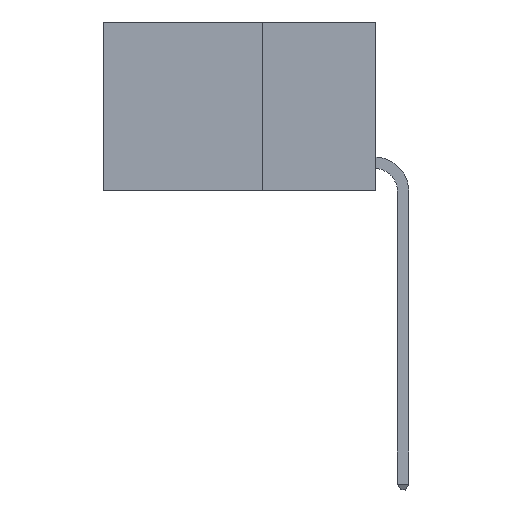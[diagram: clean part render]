
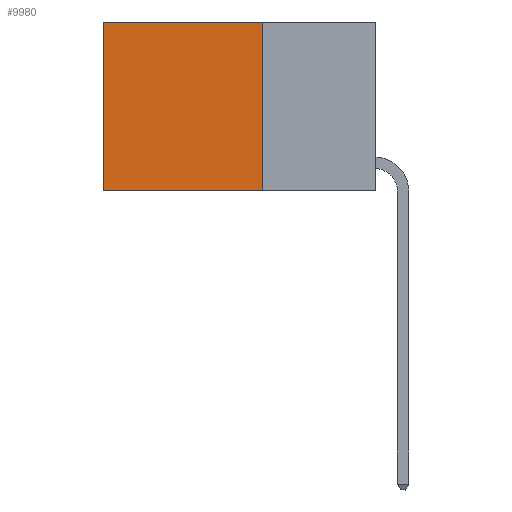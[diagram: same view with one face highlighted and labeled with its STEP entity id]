
A CAD part, left-side view. The second image highlights one B-rep face of the part: STEP entity #9980.
In plain terms, the highlighted planar face has unit normal (-1, 0, 0).
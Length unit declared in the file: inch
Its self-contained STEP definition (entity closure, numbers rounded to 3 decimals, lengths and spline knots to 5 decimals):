
#151 = ORIENTED_EDGE ( 'NONE', *, *, #3147, .F. ) ;
#350 = CARTESIAN_POINT ( 'NONE',  ( 0.2625, 0.25, -0.37 ) ) ;
#487 = VECTOR ( 'NONE', #7793, 39.37008 ) ;
#521 = CARTESIAN_POINT ( 'NONE',  ( 0.2625, 0.6, 0. ) ) ;
#723 = ORIENTED_EDGE ( 'NONE', *, *, #13557, .T. ) ;
#1414 = EDGE_LOOP ( 'NONE', ( #4210, #13328, #151, #723 ) ) ;
#2627 = CARTESIAN_POINT ( 'NONE',  ( 0.2625, 0.25, 0. ) ) ;
#3147 = EDGE_CURVE ( 'NONE', #5640, #12614, #14570, .T. ) ;
#3523 = CARTESIAN_POINT ( 'NONE',  ( 0.2625, 0.6, 0. ) ) ;
#3679 = CARTESIAN_POINT ( 'NONE',  ( 0.2625, 0.25, 0. ) ) ;
#3806 = FACE_OUTER_BOUND ( 'NONE', #1414, .T. ) ;
#3985 = CARTESIAN_POINT ( 'NONE',  ( 0.2625, 0.25, 0. ) ) ;
#4210 = ORIENTED_EDGE ( 'NONE', *, *, #14917, .T. ) ;
#4218 = DIRECTION ( 'NONE',  ( 0., 1., 0. ) ) ;
#5077 = DIRECTION ( 'NONE',  ( 0., 0., -1. ) ) ;
#5350 = DIRECTION ( 'NONE',  ( 0., 0., -1. ) ) ;
#5436 = CARTESIAN_POINT ( 'NONE',  ( 0.2625, 0.25, -0.37 ) ) ;
#5640 = VERTEX_POINT ( 'NONE', #9487 ) ;
#6260 = DIRECTION ( 'NONE',  ( 1., 0., 0. ) ) ;
#6582 = LINE ( 'NONE', #3985, #12199 ) ;
#6676 = LINE ( 'NONE', #350, #487 ) ;
#7642 = VERTEX_POINT ( 'NONE', #11876 ) ;
#7793 = DIRECTION ( 'NONE',  ( 0., 1., 0. ) ) ;
#7794 = AXIS2_PLACEMENT_3D ( 'NONE', #2627, #6260, #5077 ) ;
#9461 = VERTEX_POINT ( 'NONE', #3523 ) ;
#9487 = CARTESIAN_POINT ( 'NONE',  ( 0.2625, 0.25, 0. ) ) ;
#9980 = ADVANCED_FACE ( 'NONE', ( #3806 ), #13498, .F. ) ;
#10987 = VECTOR ( 'NONE', #5350, 39.37008 ) ;
#11264 = VECTOR ( 'NONE', #14414, 39.37008 ) ;
#11396 = LINE ( 'NONE', #521, #10987 ) ;
#11692 = EDGE_CURVE ( 'NONE', #12614, #7642, #6676, .T. ) ;
#11876 = CARTESIAN_POINT ( 'NONE',  ( 0.2625, 0.6, -0.37 ) ) ;
#12199 = VECTOR ( 'NONE', #4218, 39.37008 ) ;
#12614 = VERTEX_POINT ( 'NONE', #5436 ) ;
#13328 = ORIENTED_EDGE ( 'NONE', *, *, #11692, .F. ) ;
#13498 = PLANE ( 'NONE',  #7794 ) ;
#13557 = EDGE_CURVE ( 'NONE', #5640, #9461, #6582, .T. ) ;
#14414 = DIRECTION ( 'NONE',  ( 0., 0., -1. ) ) ;
#14570 = LINE ( 'NONE', #3679, #11264 ) ;
#14917 = EDGE_CURVE ( 'NONE', #9461, #7642, #11396, .T. ) ;
